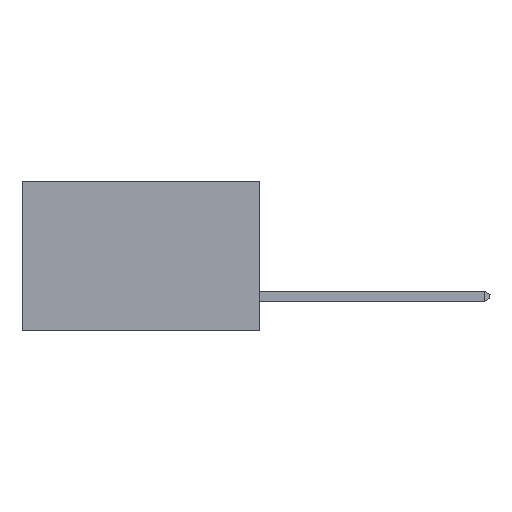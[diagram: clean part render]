
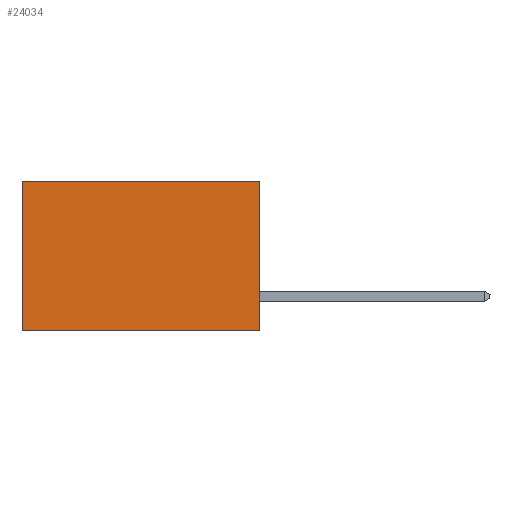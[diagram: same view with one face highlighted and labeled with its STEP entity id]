
A CAD part, left-side view. The second image highlights one B-rep face of the part: STEP entity #24034.
In plain terms, the highlighted planar face has unit normal (-1, 0, 0).
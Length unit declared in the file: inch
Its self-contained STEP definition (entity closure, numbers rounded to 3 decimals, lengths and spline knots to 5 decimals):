
#929 = ORIENTED_EDGE ( 'NONE', *, *, #2133, .F. ) ;
#1832 = CARTESIAN_POINT ( 'NONE',  ( 0.277, 0.59, -0.37 ) ) ;
#2133 = EDGE_CURVE ( 'NONE', #5126, #9819, #28610, .T. ) ;
#2526 = VERTEX_POINT ( 'NONE', #14295 ) ;
#5126 = VERTEX_POINT ( 'NONE', #29306 ) ;
#5350 = PLANE ( 'NONE',  #25525 ) ;
#7052 = VECTOR ( 'NONE', #12869, 39.37008 ) ;
#7237 = VECTOR ( 'NONE', #23917, 39.37008 ) ;
#7494 = EDGE_CURVE ( 'NONE', #9761, #5126, #24795, .T. ) ;
#9761 = VERTEX_POINT ( 'NONE', #13226 ) ;
#9819 = VERTEX_POINT ( 'NONE', #10068 ) ;
#10035 = CARTESIAN_POINT ( 'NONE',  ( 0.277, 0., -0.37 ) ) ;
#10068 = CARTESIAN_POINT ( 'NONE',  ( 0.277, 0.59, -0.37 ) ) ;
#10657 = FACE_OUTER_BOUND ( 'NONE', #28703, .T. ) ;
#10658 = ORIENTED_EDGE ( 'NONE', *, *, #10838, .T. ) ;
#10838 = EDGE_CURVE ( 'NONE', #2526, #9819, #13456, .T. ) ;
#12374 = DIRECTION ( 'NONE',  ( 1., 0., 0. ) ) ;
#12869 = DIRECTION ( 'NONE',  ( 0., 0., -1. ) ) ;
#12931 = CARTESIAN_POINT ( 'NONE',  ( 0.277, 0., -0.37 ) ) ;
#13119 = EDGE_CURVE ( 'NONE', #9761, #2526, #17711, .T. ) ;
#13226 = CARTESIAN_POINT ( 'NONE',  ( 0.277, 0., 0. ) ) ;
#13456 = LINE ( 'NONE', #1832, #7237 ) ;
#14295 = CARTESIAN_POINT ( 'NONE',  ( 0.277, 0.59, 0. ) ) ;
#14868 = CARTESIAN_POINT ( 'NONE',  ( 0.277, 0., -0.37 ) ) ;
#17711 = LINE ( 'NONE', #21420, #29265 ) ;
#19200 = DIRECTION ( 'NONE',  ( 0., 1., 0. ) ) ;
#19674 = ORIENTED_EDGE ( 'NONE', *, *, #7494, .F. ) ;
#21420 = CARTESIAN_POINT ( 'NONE',  ( 0.277, 0., 0. ) ) ;
#23189 = VECTOR ( 'NONE', #24026, 39.37008 ) ;
#23917 = DIRECTION ( 'NONE',  ( 0., 0., -1. ) ) ;
#24026 = DIRECTION ( 'NONE',  ( 0., 1., 0. ) ) ;
#24034 = ADVANCED_FACE ( 'NONE', ( #10657 ), #5350, .F. ) ;
#24795 = LINE ( 'NONE', #12931, #7052 ) ;
#25525 = AXIS2_PLACEMENT_3D ( 'NONE', #10035, #12374, #28514 ) ;
#28514 = DIRECTION ( 'NONE',  ( 0., 0., -1. ) ) ;
#28610 = LINE ( 'NONE', #14868, #23189 ) ;
#28703 = EDGE_LOOP ( 'NONE', ( #10658, #929, #19674, #29635 ) ) ;
#29265 = VECTOR ( 'NONE', #19200, 39.37008 ) ;
#29306 = CARTESIAN_POINT ( 'NONE',  ( 0.277, 0., -0.37 ) ) ;
#29635 = ORIENTED_EDGE ( 'NONE', *, *, #13119, .T. ) ;
